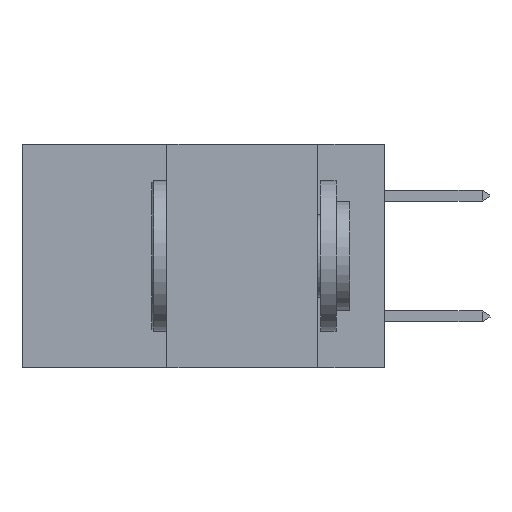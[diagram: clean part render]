
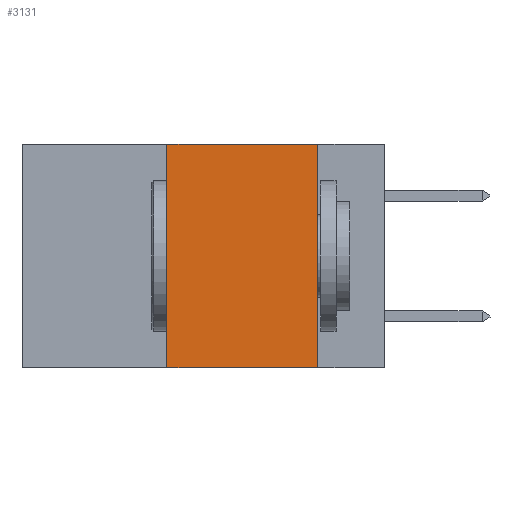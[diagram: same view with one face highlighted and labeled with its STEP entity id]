
A CAD part, left-side view. The second image highlights one B-rep face of the part: STEP entity #3131.
In plain terms, the highlighted planar face has unit normal (-1, 0, 0).
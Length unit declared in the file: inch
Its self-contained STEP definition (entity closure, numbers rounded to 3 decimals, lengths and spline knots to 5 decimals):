
#172 = CARTESIAN_POINT ( 'NONE',  ( 0., 0.6, 0. ) ) ;
#381 = DIRECTION ( 'NONE',  ( 0., 0., -1. ) ) ;
#602 = LINE ( 'NONE', #172, #13477 ) ;
#626 = DIRECTION ( 'NONE',  ( 0., -1., 0. ) ) ;
#868 = VECTOR ( 'NONE', #626, 39.37008 ) ;
#1123 = EDGE_CURVE ( 'NONE', #8410, #7007, #602, .T. ) ;
#1541 = CARTESIAN_POINT ( 'NONE',  ( 0., 0.6, 0. ) ) ;
#2257 = ORIENTED_EDGE ( 'NONE', *, *, #6322, .F. ) ;
#2263 = ORIENTED_EDGE ( 'NONE', *, *, #13647, .T. ) ;
#2624 = FACE_OUTER_BOUND ( 'NONE', #12353, .T. ) ;
#3014 = AXIS2_PLACEMENT_3D ( 'NONE', #1541, #13681, #381 ) ;
#3131 = ADVANCED_FACE ( 'NONE', ( #2624 ), #10010, .F. ) ;
#3307 = LINE ( 'NONE', #6178, #868 ) ;
#3734 = VECTOR ( 'NONE', #9529, 39.37008 ) ;
#4123 = EDGE_CURVE ( 'NONE', #13020, #8410, #9540, .T. ) ;
#5519 = VECTOR ( 'NONE', #10982, 39.37008 ) ;
#6178 = CARTESIAN_POINT ( 'NONE',  ( 0., 0.6, -0.37 ) ) ;
#6322 = EDGE_CURVE ( 'NONE', #7007, #7087, #11234, .T. ) ;
#6758 = ORIENTED_EDGE ( 'NONE', *, *, #4123, .F. ) ;
#6851 = CARTESIAN_POINT ( 'NONE',  ( 0., 0.11, 0. ) ) ;
#7007 = VERTEX_POINT ( 'NONE', #6851 ) ;
#7087 = VERTEX_POINT ( 'NONE', #11645 ) ;
#8262 = CARTESIAN_POINT ( 'NONE',  ( 0., 0.36, 0. ) ) ;
#8410 = VERTEX_POINT ( 'NONE', #8262 ) ;
#9277 = ORIENTED_EDGE ( 'NONE', *, *, #1123, .F. ) ;
#9444 = CARTESIAN_POINT ( 'NONE',  ( 0., 0.11, 0. ) ) ;
#9529 = DIRECTION ( 'NONE',  ( 0., 0., -1. ) ) ;
#9540 = LINE ( 'NONE', #9975, #5519 ) ;
#9975 = CARTESIAN_POINT ( 'NONE',  ( 0., 0.36, 0. ) ) ;
#10010 = PLANE ( 'NONE',  #3014 ) ;
#10048 = DIRECTION ( 'NONE',  ( 0., -1., 0. ) ) ;
#10982 = DIRECTION ( 'NONE',  ( 0., 0., 1. ) ) ;
#11234 = LINE ( 'NONE', #9444, #3734 ) ;
#11645 = CARTESIAN_POINT ( 'NONE',  ( 0., 0.11, -0.37 ) ) ;
#12353 = EDGE_LOOP ( 'NONE', ( #2257, #9277, #6758, #2263 ) ) ;
#13020 = VERTEX_POINT ( 'NONE', #13737 ) ;
#13477 = VECTOR ( 'NONE', #10048, 39.37008 ) ;
#13647 = EDGE_CURVE ( 'NONE', #13020, #7087, #3307, .T. ) ;
#13681 = DIRECTION ( 'NONE',  ( 1., 0., 0. ) ) ;
#13737 = CARTESIAN_POINT ( 'NONE',  ( 0., 0.36, -0.37 ) ) ;
